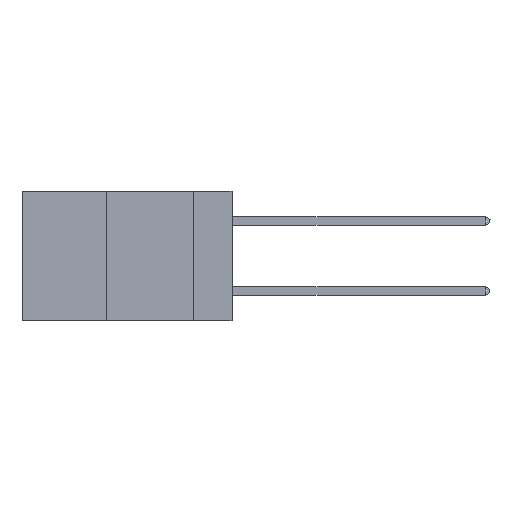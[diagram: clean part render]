
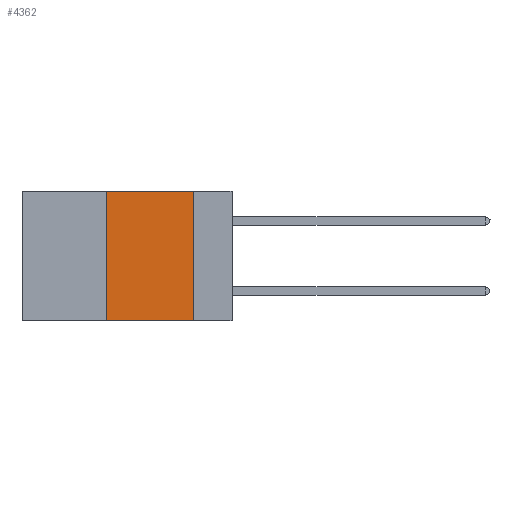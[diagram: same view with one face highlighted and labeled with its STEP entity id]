
A CAD part, left-side view. The second image highlights one B-rep face of the part: STEP entity #4362.
In plain terms, the highlighted planar face has unit normal (-1, 0, 0).
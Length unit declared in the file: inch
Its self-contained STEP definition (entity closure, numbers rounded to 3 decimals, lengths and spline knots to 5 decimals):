
#168 = VECTOR ( 'NONE', #12047, 39.37008 ) ;
#405 = CARTESIAN_POINT ( 'NONE',  ( 0., 0.6, 0. ) ) ;
#598 = EDGE_CURVE ( 'NONE', #9634, #2043, #10408, .T. ) ;
#729 = DIRECTION ( 'NONE',  ( 0., 0., 1. ) ) ;
#1416 = VECTOR ( 'NONE', #11388, 39.37008 ) ;
#1767 = LINE ( 'NONE', #5593, #9587 ) ;
#2043 = VERTEX_POINT ( 'NONE', #8041 ) ;
#2206 = FACE_OUTER_BOUND ( 'NONE', #3423, .T. ) ;
#2361 = VERTEX_POINT ( 'NONE', #3910 ) ;
#3423 = EDGE_LOOP ( 'NONE', ( #10274, #7612, #9797, #10364 ) ) ;
#3910 = CARTESIAN_POINT ( 'NONE',  ( 0., 0.36, 0. ) ) ;
#4215 = AXIS2_PLACEMENT_3D ( 'NONE', #8219, #5188, #9124 ) ;
#4249 = LINE ( 'NONE', #8254, #168 ) ;
#4269 = PLANE ( 'NONE',  #4215 ) ;
#4362 = ADVANCED_FACE ( 'NONE', ( #2206 ), #4269, .F. ) ;
#5188 = DIRECTION ( 'NONE',  ( 1., 0., 0. ) ) ;
#5190 = EDGE_CURVE ( 'NONE', #5944, #2043, #4249, .T. ) ;
#5423 = VECTOR ( 'NONE', #10470, 39.37008 ) ;
#5593 = CARTESIAN_POINT ( 'NONE',  ( 0., 0.36, 0. ) ) ;
#5747 = EDGE_CURVE ( 'NONE', #2361, #5944, #6311, .T. ) ;
#5944 = VERTEX_POINT ( 'NONE', #9763 ) ;
#6311 = LINE ( 'NONE', #405, #1416 ) ;
#7612 = ORIENTED_EDGE ( 'NONE', *, *, #5747, .F. ) ;
#8041 = CARTESIAN_POINT ( 'NONE',  ( 0., 0.11, -0.37 ) ) ;
#8219 = CARTESIAN_POINT ( 'NONE',  ( 0., 0.6, 0. ) ) ;
#8254 = CARTESIAN_POINT ( 'NONE',  ( 0., 0.11, 0. ) ) ;
#8675 = CARTESIAN_POINT ( 'NONE',  ( 0., 0.6, -0.37 ) ) ;
#9124 = DIRECTION ( 'NONE',  ( 0., 0., -1. ) ) ;
#9587 = VECTOR ( 'NONE', #729, 39.37008 ) ;
#9634 = VERTEX_POINT ( 'NONE', #12309 ) ;
#9763 = CARTESIAN_POINT ( 'NONE',  ( 0., 0.11, 0. ) ) ;
#9797 = ORIENTED_EDGE ( 'NONE', *, *, #11616, .F. ) ;
#10274 = ORIENTED_EDGE ( 'NONE', *, *, #5190, .F. ) ;
#10364 = ORIENTED_EDGE ( 'NONE', *, *, #598, .T. ) ;
#10408 = LINE ( 'NONE', #8675, #5423 ) ;
#10470 = DIRECTION ( 'NONE',  ( 0., -1., 0. ) ) ;
#11388 = DIRECTION ( 'NONE',  ( 0., -1., 0. ) ) ;
#11616 = EDGE_CURVE ( 'NONE', #9634, #2361, #1767, .T. ) ;
#12047 = DIRECTION ( 'NONE',  ( 0., 0., -1. ) ) ;
#12309 = CARTESIAN_POINT ( 'NONE',  ( 0., 0.36, -0.37 ) ) ;
